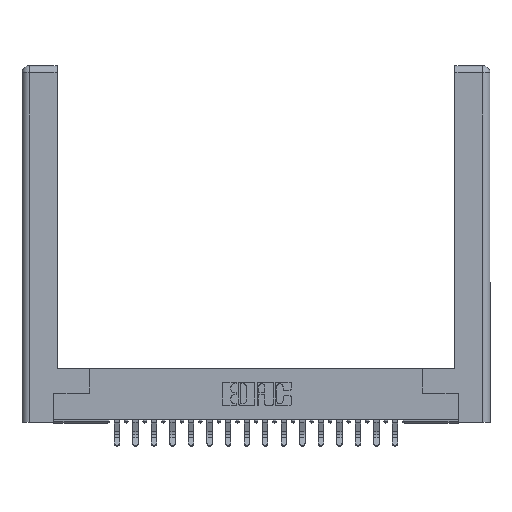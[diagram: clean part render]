
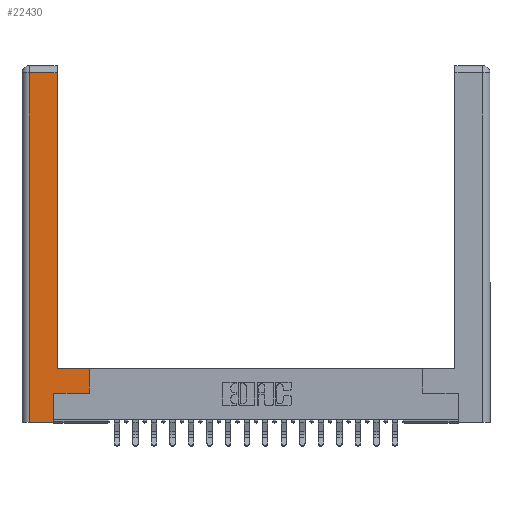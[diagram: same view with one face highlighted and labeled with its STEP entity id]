
A CAD part, top view. The second image highlights one B-rep face of the part: STEP entity #22430.
In plain terms, the highlighted planar face has unit normal (0, 0, 1).
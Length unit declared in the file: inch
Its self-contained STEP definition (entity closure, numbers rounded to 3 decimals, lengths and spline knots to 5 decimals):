
#486 = DIRECTION ( 'NONE',  ( -1., 0., 0. ) ) ;
#646 = CARTESIAN_POINT ( 'NONE',  ( 0.565, 0.245, 0. ) ) ;
#819 = VECTOR ( 'NONE', #486, 39.37008 ) ;
#1129 = VERTEX_POINT ( 'NONE', #15258 ) ;
#2229 = VECTOR ( 'NONE', #15381, 39.37008 ) ;
#2654 = LINE ( 'NONE', #14584, #16958 ) ;
#2908 = EDGE_CURVE ( 'NONE', #9249, #22894, #3337, .T. ) ;
#2993 = DIRECTION ( 'NONE',  ( 1., 0., 0. ) ) ;
#3314 = DIRECTION ( 'NONE',  ( 0., 0., -1. ) ) ;
#3337 = LINE ( 'NONE', #21357, #14901 ) ;
#3338 = LINE ( 'NONE', #11558, #2229 ) ;
#3396 = LINE ( 'NONE', #17039, #21742 ) ;
#3652 = CARTESIAN_POINT ( 'NONE',  ( 0.295, 0.45, 0. ) ) ;
#4400 = DIRECTION ( 'NONE',  ( 0., 1., 0. ) ) ;
#4587 = DIRECTION ( 'NONE',  ( 0., 1., 0. ) ) ;
#4643 = ORIENTED_EDGE ( 'NONE', *, *, #17062, .T. ) ;
#4655 = FACE_OUTER_BOUND ( 'NONE', #17686, .T. ) ;
#5046 = PLANE ( 'NONE',  #18746 ) ;
#5131 = DIRECTION ( 'NONE',  ( -1., 0., 0. ) ) ;
#5523 = ORIENTED_EDGE ( 'NONE', *, *, #12483, .T. ) ;
#5699 = ORIENTED_EDGE ( 'NONE', *, *, #18875, .T. ) ;
#6822 = CARTESIAN_POINT ( 'NONE',  ( 0., 0., 0. ) ) ;
#7273 = CARTESIAN_POINT ( 'NONE',  ( 0.295, 2.94, 0. ) ) ;
#7472 = EDGE_CURVE ( 'NONE', #18450, #8588, #3396, .T. ) ;
#8134 = CARTESIAN_POINT ( 'NONE',  ( 0.565, 0.45, 0. ) ) ;
#8588 = VERTEX_POINT ( 'NONE', #7273 ) ;
#8681 = CARTESIAN_POINT ( 'NONE',  ( 0.265, 0., 0. ) ) ;
#9249 = VERTEX_POINT ( 'NONE', #16102 ) ;
#9665 = LINE ( 'NONE', #8134, #23224 ) ;
#9836 = LINE ( 'NONE', #18368, #819 ) ;
#10017 = ORIENTED_EDGE ( 'NONE', *, *, #7472, .T. ) ;
#10120 = VERTEX_POINT ( 'NONE', #18393 ) ;
#10573 = CARTESIAN_POINT ( 'NONE',  ( 0.265, 0.245, 0. ) ) ;
#11149 = ORIENTED_EDGE ( 'NONE', *, *, #19664, .T. ) ;
#11178 = EDGE_CURVE ( 'NONE', #22894, #22884, #13943, .T. ) ;
#11198 = DIRECTION ( 'NONE',  ( 0., -1., 0. ) ) ;
#11558 = CARTESIAN_POINT ( 'NONE',  ( 0.565, 0.245, 0. ) ) ;
#12483 = EDGE_CURVE ( 'NONE', #22318, #1129, #9665, .T. ) ;
#12530 = ORIENTED_EDGE ( 'NONE', *, *, #11178, .T. ) ;
#12540 = CARTESIAN_POINT ( 'NONE',  ( 0.295, 0.45, 0. ) ) ;
#13594 = LINE ( 'NONE', #3652, #16680 ) ;
#13943 = LINE ( 'NONE', #16840, #17314 ) ;
#14584 = CARTESIAN_POINT ( 'NONE',  ( 0.0615, 0., 0. ) ) ;
#14901 = VECTOR ( 'NONE', #2993, 39.37008 ) ;
#14908 = ORIENTED_EDGE ( 'NONE', *, *, #2908, .T. ) ;
#15258 = CARTESIAN_POINT ( 'NONE',  ( 0.565, 0.45, 0. ) ) ;
#15381 = DIRECTION ( 'NONE',  ( 1., 0., 0. ) ) ;
#16102 = CARTESIAN_POINT ( 'NONE',  ( 0.0615, 0., 0. ) ) ;
#16212 = DIRECTION ( 'NONE',  ( -1., 0., 0. ) ) ;
#16680 = VECTOR ( 'NONE', #16212, 39.37008 ) ;
#16840 = CARTESIAN_POINT ( 'NONE',  ( 0.265, 0.245, 0. ) ) ;
#16958 = VECTOR ( 'NONE', #11198, 39.37008 ) ;
#17039 = CARTESIAN_POINT ( 'NONE',  ( 0.295, 3., 0. ) ) ;
#17062 = EDGE_CURVE ( 'NONE', #1129, #18450, #13594, .T. ) ;
#17314 = VECTOR ( 'NONE', #4587, 39.37008 ) ;
#17686 = EDGE_LOOP ( 'NONE', ( #10017, #5699, #19762, #14908, #12530, #11149, #5523, #4643 ) ) ;
#18368 = CARTESIAN_POINT ( 'NONE',  ( 0.0615, 2.94, 0. ) ) ;
#18393 = CARTESIAN_POINT ( 'NONE',  ( 0.0615, 2.94, 0. ) ) ;
#18450 = VERTEX_POINT ( 'NONE', #12540 ) ;
#18746 = AXIS2_PLACEMENT_3D ( 'NONE', #6822, #3314, #5131 ) ;
#18875 = EDGE_CURVE ( 'NONE', #8588, #10120, #9836, .T. ) ;
#19664 = EDGE_CURVE ( 'NONE', #22884, #22318, #3338, .T. ) ;
#19762 = ORIENTED_EDGE ( 'NONE', *, *, #23226, .T. ) ;
#20766 = DIRECTION ( 'NONE',  ( 0., 1., 0. ) ) ;
#21357 = CARTESIAN_POINT ( 'NONE',  ( 0.265, 0., 0. ) ) ;
#21742 = VECTOR ( 'NONE', #4400, 39.37008 ) ;
#22318 = VERTEX_POINT ( 'NONE', #646 ) ;
#22430 = ADVANCED_FACE ( 'NONE', ( #4655 ), #5046, .F. ) ;
#22884 = VERTEX_POINT ( 'NONE', #10573 ) ;
#22894 = VERTEX_POINT ( 'NONE', #8681 ) ;
#23224 = VECTOR ( 'NONE', #20766, 39.37008 ) ;
#23226 = EDGE_CURVE ( 'NONE', #10120, #9249, #2654, .T. ) ;
